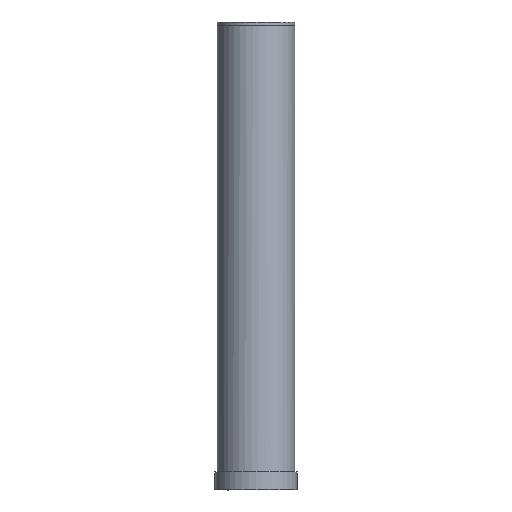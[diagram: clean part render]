
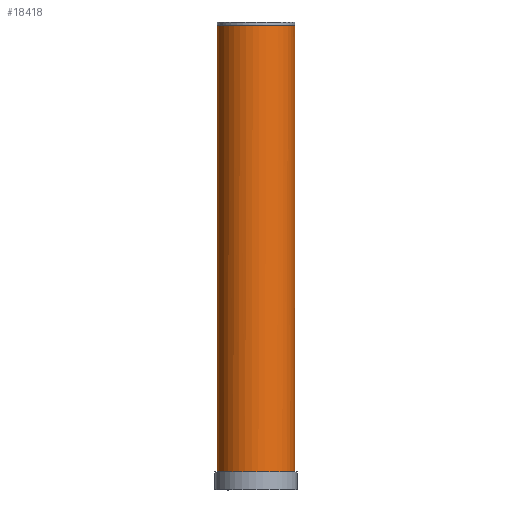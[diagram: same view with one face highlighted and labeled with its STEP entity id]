
A CAD part, front view. The second image highlights one B-rep face of the part: STEP entity #18418.
In plain terms, the highlighted cylindrical face has radius 17.513 mm (diameter 35.027 mm), a full revolution.
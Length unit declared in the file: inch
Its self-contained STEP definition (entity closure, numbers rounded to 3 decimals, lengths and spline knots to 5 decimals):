
#258 = ORIENTED_EDGE ( 'NONE', *, *, #19611, .F. ) ;
#580 = CARTESIAN_POINT ( 'NONE',  ( 0.05706, 0.68714, 7.92684 ) ) ;
#653 = CARTESIAN_POINT ( 'NONE',  ( -0.03182, 0.68877, 7.89989 ) ) ;
#1007 = LINE ( 'NONE', #22316, #9767 ) ;
#1189 = VERTEX_POINT ( 'NONE', #8208 ) ;
#1371 = DIRECTION ( 'NONE',  ( 0., 0., -1. ) ) ;
#1600 = ORIENTED_EDGE ( 'NONE', *, *, #21114, .F. ) ;
#2002 = VERTEX_POINT ( 'NONE', #8195 ) ;
#2332 = CARTESIAN_POINT ( 'NONE',  ( 0.05051, 0.68765, 7.91629 ) ) ;
#2406 = CARTESIAN_POINT ( 'NONE',  ( -0.0419, 0.68823, 7.90711 ) ) ;
#2601 = VERTEX_POINT ( 'NONE', #12698 ) ;
#3951 = EDGE_LOOP ( 'NONE', ( #1600, #258, #10052, #18072 ) ) ;
#3976 = EDGE_CURVE ( 'NONE', #2601, #2601, #6560, .T. ) ;
#4095 = CARTESIAN_POINT ( 'NONE',  ( 0.03905, 0.68842, 7.90424 ) ) ;
#4175 = CARTESIAN_POINT ( 'NONE',  ( -0.05046, 0.68765, 7.91624 ) ) ;
#5820 = DIRECTION ( 'NONE',  ( 0., 0., 1. ) ) ;
#5839 = CARTESIAN_POINT ( 'NONE',  ( 0.01669, 0.68934, 7.89318 ) ) ;
#5917 = CARTESIAN_POINT ( 'NONE',  ( -0.05706, 0.68714, 7.92682 ) ) ;
#6013 = CARTESIAN_POINT ( 'NONE',  ( -0.0635, 0.68657, 8.035 ) ) ;
#6424 = VERTEX_POINT ( 'NONE', #11241 ) ;
#6560 = CIRCLE ( 'NONE', #7567, 0.6895 ) ;
#7567 = AXIS2_PLACEMENT_3D ( 'NONE', #19702, #9227, #21453 ) ;
#7618 = CARTESIAN_POINT ( 'NONE',  ( -0.0041, 0.6895, 7.8915 ) ) ;
#7696 = CARTESIAN_POINT ( 'NONE',  ( -0.0635, 0.68657, 7.94661 ) ) ;
#8195 = CARTESIAN_POINT ( 'NONE',  ( -0.0635, 0.68657, 7.955 ) ) ;
#8208 = CARTESIAN_POINT ( 'NONE',  ( 0.0635, 0.68657, 7.955 ) ) ;
#8879 = B_SPLINE_CURVE_WITH_KNOTS ( 'NONE', 3,
 ( #14505, #19693, #9299, #21520, #11051, #580, #12811, #2332, #14586, #4095, #16360, #5839, #18098, #7618, #19851, #9377, #21598, #11120, #653, #12893, #2406, #14657, #4175, #16435, #5917, #18166, #7696, #19917 ),
 .UNSPECIFIED., .F., .F.,
 ( 4, 2, 2, 2, 2, 2, 2, 2, 2, 2, 2, 2, 2, 4 ),
 ( 0., 0.00032, 0.00063, 0.00095, 0.00126, 0.00189, 0.00252, 0.00284, 0.00315, 0.00347, 0.00378, 0.0041, 0.00441, 0.00504 ),
 .UNSPECIFIED. ) ;
#9227 = DIRECTION ( 'NONE',  ( 0., 0., 1. ) ) ;
#9299 = CARTESIAN_POINT ( 'NONE',  ( 0.06309, 0.68661, 7.94668 ) ) ;
#9377 = CARTESIAN_POINT ( 'NONE',  ( -0.01645, 0.68932, 7.89353 ) ) ;
#9542 = VERTEX_POINT ( 'NONE', #6013 ) ;
#9572 = EDGE_CURVE ( 'NONE', #2002, #9542, #22359, .T. ) ;
#9767 = VECTOR ( 'NONE', #1371, 39.37008 ) ;
#10052 = ORIENTED_EDGE ( 'NONE', *, *, #9572, .F. ) ;
#10252 = AXIS2_PLACEMENT_3D ( 'NONE', #21872, #11393, #16615 ) ;
#11051 = CARTESIAN_POINT ( 'NONE',  ( 0.06025, 0.68686, 7.93453 ) ) ;
#11120 = CARTESIAN_POINT ( 'NONE',  ( -0.0281, 0.68894, 7.8979 ) ) ;
#11241 = CARTESIAN_POINT ( 'NONE',  ( 0.0635, 0.68657, 8.035 ) ) ;
#11393 = DIRECTION ( 'NONE',  ( 0., 0., -1. ) ) ;
#12698 = CARTESIAN_POINT ( 'NONE',  ( 0.6895, 0., 0. ) ) ;
#12808 = EDGE_LOOP ( 'NONE', ( #21511 ) ) ;
#12811 = CARTESIAN_POINT ( 'NONE',  ( 0.05511, 0.6873, 7.92319 ) ) ;
#12893 = CARTESIAN_POINT ( 'NONE',  ( -0.0387, 0.68842, 7.90448 ) ) ;
#12959 = EDGE_CURVE ( 'NONE', #1189, #2002, #8879, .T. ) ;
#13934 = FACE_OUTER_BOUND ( 'NONE', #3951, .T. ) ;
#14493 = FACE_OUTER_BOUND ( 'NONE', #12808, .T. ) ;
#14505 = CARTESIAN_POINT ( 'NONE',  ( 0.0635, 0.68657, 7.955 ) ) ;
#14586 = CARTESIAN_POINT ( 'NONE',  ( 0.04783, 0.68785, 7.91302 ) ) ;
#14657 = CARTESIAN_POINT ( 'NONE',  ( -0.04784, 0.68785, 7.91303 ) ) ;
#15847 = CIRCLE ( 'NONE', #16454, 0.6895 ) ;
#16341 = CARTESIAN_POINT ( 'NONE',  ( 0., 0., 8.035 ) ) ;
#16360 = CARTESIAN_POINT ( 'NONE',  ( 0.03197, 0.6888, 7.89951 ) ) ;
#16435 = CARTESIAN_POINT ( 'NONE',  ( -0.05507, 0.6873, 7.92311 ) ) ;
#16454 = AXIS2_PLACEMENT_3D ( 'NONE', #16341, #5820, #18075 ) ;
#16615 = DIRECTION ( 'NONE',  ( -1., 0., 0. ) ) ;
#16664 = CARTESIAN_POINT ( 'NONE',  ( -0.0635, 0.68657, 8.035 ) ) ;
#17183 = VECTOR ( 'NONE', #18413, 39.37008 ) ;
#18072 = ORIENTED_EDGE ( 'NONE', *, *, #12959, .F. ) ;
#18075 = DIRECTION ( 'NONE',  ( 1., 0., 0. ) ) ;
#18098 = CARTESIAN_POINT ( 'NONE',  ( 0.00833, 0.6895, 7.89151 ) ) ;
#18166 = CARTESIAN_POINT ( 'NONE',  ( -0.06184, 0.68673, 7.93835 ) ) ;
#18413 = DIRECTION ( 'NONE',  ( 0., 0., 1. ) ) ;
#18418 = ADVANCED_FACE ( 'NONE', ( #14493, #13934 ), #22681, .T. ) ;
#19611 = EDGE_CURVE ( 'NONE', #9542, #6424, #15847, .T. ) ;
#19693 = CARTESIAN_POINT ( 'NONE',  ( 0.0635, 0.68657, 7.9508 ) ) ;
#19702 = CARTESIAN_POINT ( 'NONE',  ( 0., 0., 0. ) ) ;
#19851 = CARTESIAN_POINT ( 'NONE',  ( -0.00831, 0.68946, 7.89191 ) ) ;
#19917 = CARTESIAN_POINT ( 'NONE',  ( -0.0635, 0.68657, 7.955 ) ) ;
#21114 = EDGE_CURVE ( 'NONE', #6424, #1189, #1007, .T. ) ;
#21453 = DIRECTION ( 'NONE',  ( 1., 0., 0. ) ) ;
#21511 = ORIENTED_EDGE ( 'NONE', *, *, #3976, .T. ) ;
#21520 = CARTESIAN_POINT ( 'NONE',  ( 0.06147, 0.68675, 7.93856 ) ) ;
#21598 = CARTESIAN_POINT ( 'NONE',  ( -0.02041, 0.68921, 7.89473 ) ) ;
#21872 = CARTESIAN_POINT ( 'NONE',  ( 0., 0., 8.035 ) ) ;
#22316 = CARTESIAN_POINT ( 'NONE',  ( 0.0635, 0.68657, 8.035 ) ) ;
#22359 = LINE ( 'NONE', #16664, #17183 ) ;
#22681 = CYLINDRICAL_SURFACE ( 'NONE', #10252, 0.6895 ) ;
